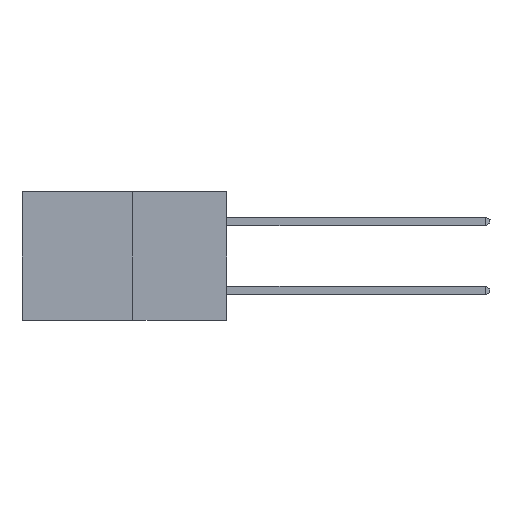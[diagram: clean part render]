
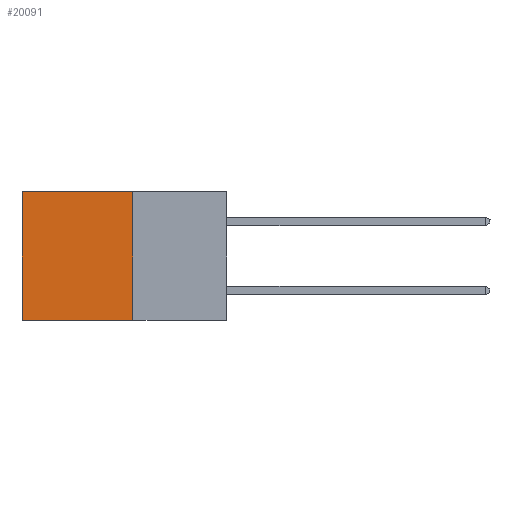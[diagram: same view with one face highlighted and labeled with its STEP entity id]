
A CAD part, left-side view. The second image highlights one B-rep face of the part: STEP entity #20091.
In plain terms, the highlighted planar face has unit normal (-1, 0, 0).
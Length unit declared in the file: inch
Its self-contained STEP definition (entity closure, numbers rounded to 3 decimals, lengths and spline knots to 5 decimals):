
#385 = LINE ( 'NONE', #21704, #33636 ) ;
#1006 = EDGE_LOOP ( 'NONE', ( #12099, #7142, #27497, #19647 ) ) ;
#1072 = PLANE ( 'NONE',  #14344 ) ;
#1413 = VERTEX_POINT ( 'NONE', #17249 ) ;
#3751 = DIRECTION ( 'NONE',  ( 0., 0., -1. ) ) ;
#5804 = DIRECTION ( 'NONE',  ( 0., 1., 0. ) ) ;
#7142 = ORIENTED_EDGE ( 'NONE', *, *, #25254, .F. ) ;
#8014 = DIRECTION ( 'NONE',  ( 0., 0., -1. ) ) ;
#8738 = EDGE_CURVE ( 'NONE', #23936, #11417, #385, .T. ) ;
#9679 = CARTESIAN_POINT ( 'NONE',  ( 0.277, 0.27, 0. ) ) ;
#10201 = LINE ( 'NONE', #32696, #23482 ) ;
#11417 = VERTEX_POINT ( 'NONE', #24716 ) ;
#11788 = LINE ( 'NONE', #30961, #18045 ) ;
#12099 = ORIENTED_EDGE ( 'NONE', *, *, #19852, .T. ) ;
#14344 = AXIS2_PLACEMENT_3D ( 'NONE', #29978, #19656, #3751 ) ;
#16549 = VERTEX_POINT ( 'NONE', #25979 ) ;
#17168 = DIRECTION ( 'NONE',  ( 0., 0., -1. ) ) ;
#17249 = CARTESIAN_POINT ( 'NONE',  ( 0.277, 0.59, -0.37 ) ) ;
#18045 = VECTOR ( 'NONE', #33509, 39.37008 ) ;
#18129 = LINE ( 'NONE', #18628, #31137 ) ;
#18628 = CARTESIAN_POINT ( 'NONE',  ( 0.277, 0.59, -0.37 ) ) ;
#19647 = ORIENTED_EDGE ( 'NONE', *, *, #8738, .T. ) ;
#19656 = DIRECTION ( 'NONE',  ( 1., 0., 0. ) ) ;
#19852 = EDGE_CURVE ( 'NONE', #11417, #1413, #18129, .T. ) ;
#20091 = ADVANCED_FACE ( 'NONE', ( #30723 ), #1072, .F. ) ;
#21704 = CARTESIAN_POINT ( 'NONE',  ( 0.277, 0.27, 0. ) ) ;
#23482 = VECTOR ( 'NONE', #17168, 39.37008 ) ;
#23936 = VERTEX_POINT ( 'NONE', #9679 ) ;
#24716 = CARTESIAN_POINT ( 'NONE',  ( 0.277, 0.59, 0. ) ) ;
#25254 = EDGE_CURVE ( 'NONE', #16549, #1413, #11788, .T. ) ;
#25979 = CARTESIAN_POINT ( 'NONE',  ( 0.277, 0.27, -0.37 ) ) ;
#27497 = ORIENTED_EDGE ( 'NONE', *, *, #29159, .F. ) ;
#29159 = EDGE_CURVE ( 'NONE', #23936, #16549, #10201, .T. ) ;
#29978 = CARTESIAN_POINT ( 'NONE',  ( 0.277, 0.27, -0.37 ) ) ;
#30723 = FACE_OUTER_BOUND ( 'NONE', #1006, .T. ) ;
#30961 = CARTESIAN_POINT ( 'NONE',  ( 0.277, 0.27, -0.37 ) ) ;
#31137 = VECTOR ( 'NONE', #8014, 39.37008 ) ;
#32696 = CARTESIAN_POINT ( 'NONE',  ( 0.277, 0.27, -0.37 ) ) ;
#33509 = DIRECTION ( 'NONE',  ( 0., 1., 0. ) ) ;
#33636 = VECTOR ( 'NONE', #5804, 39.37008 ) ;
